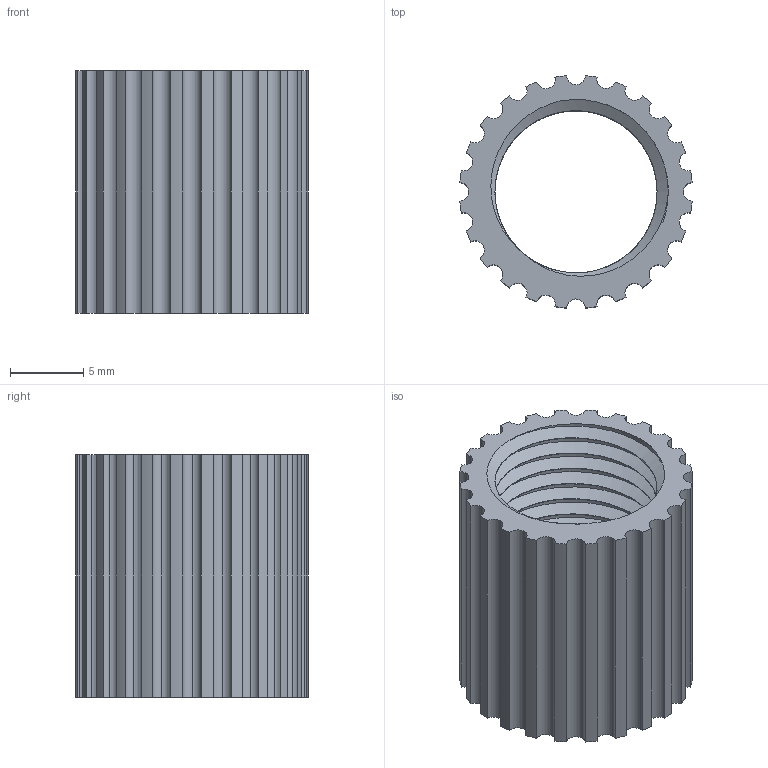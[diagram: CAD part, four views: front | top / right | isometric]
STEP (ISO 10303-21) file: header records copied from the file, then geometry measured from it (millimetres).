
FILE_DESCRIPTION (( 'STEP AP203' ), '1' );
FILE_NAME ('AF-HF-LR-PRT-008-STEP.STEP', '2020-10-04T16:15:35', ( '' ), ( '' ), 'SwSTEP 2.0', 'SolidWorks 2018', '' );
FILE_SCHEMA (( 'CONFIG_CONTROL_DESIGN' ));
Length unit declared in the file: inch
Products named in the file (1): AF-HF-LR-PRT-008-STEP
Bounding box: 15.82 x 15.82 x 16.51 mm (x, y, z)
Volume: 1143 mm3; surface area: 2123.9 mm2
Topology: 1 solids, 1 shells, 85 faces, 247 edges, 164 vertices
Faces by surface type: cylinder 78, plane 4, bspline 3
Entity records: 6860 total; most frequent: CARTESIAN_POINT 4522, DIRECTION 495, ORIENTED_EDGE 494, EDGE_CURVE 247, AXIS2_PLACEMENT_3D 209, VERTEX_POINT 164, CIRCLE 126, EDGE_LOOP 87
